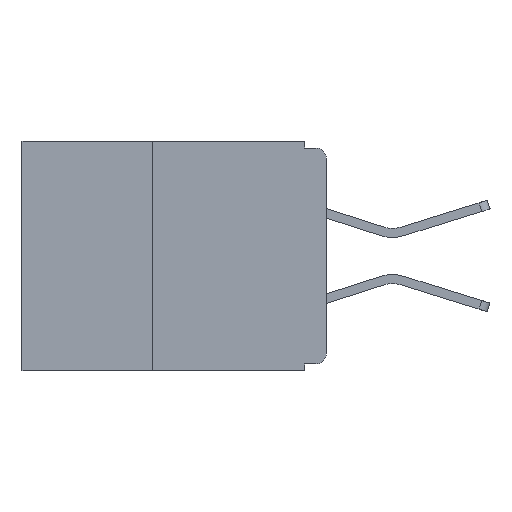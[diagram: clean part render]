
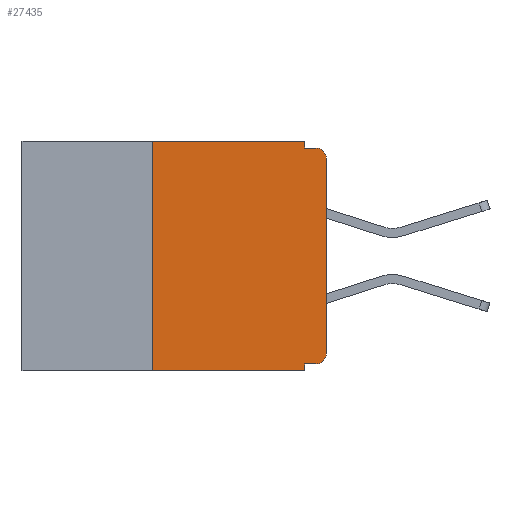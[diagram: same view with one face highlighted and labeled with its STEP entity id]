
A CAD part, left-side view. The second image highlights one B-rep face of the part: STEP entity #27435.
In plain terms, the highlighted planar face has unit normal (-1, 0, 0).
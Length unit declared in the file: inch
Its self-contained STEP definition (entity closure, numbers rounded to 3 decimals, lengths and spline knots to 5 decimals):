
#333 = VECTOR ( 'NONE', #11495, 39.37008 ) ;
#669 = CARTESIAN_POINT ( 'NONE',  ( 0., 0.031, -0.33 ) ) ;
#891 = LINE ( 'NONE', #5456, #17757 ) ;
#1060 = DIRECTION ( 'NONE',  ( 0., 0., -1. ) ) ;
#1680 = ORIENTED_EDGE ( 'NONE', *, *, #9738, .T. ) ;
#1788 = DIRECTION ( 'NONE',  ( 1., 0., 0. ) ) ;
#2608 = LINE ( 'NONE', #24491, #7786 ) ;
#2718 = ORIENTED_EDGE ( 'NONE', *, *, #19798, .T. ) ;
#3532 = DIRECTION ( 'NONE',  ( -1., 0., 0. ) ) ;
#3645 = LINE ( 'NONE', #22885, #8799 ) ;
#3854 = EDGE_CURVE ( 'NONE', #20469, #16692, #12098, .T. ) ;
#4030 = VECTOR ( 'NONE', #11167, 39.37008 ) ;
#4216 = VERTEX_POINT ( 'NONE', #9348 ) ;
#4595 = CARTESIAN_POINT ( 'NONE',  ( 0., 0., -0.01 ) ) ;
#4618 = EDGE_CURVE ( 'NONE', #8001, #8071, #25678, .T. ) ;
#4669 = VECTOR ( 'NONE', #8589, 39.37008 ) ;
#5195 = DIRECTION ( 'NONE',  ( 0., 0., 1. ) ) ;
#5456 = CARTESIAN_POINT ( 'NONE',  ( 0., 0.031, 0. ) ) ;
#5516 = ORIENTED_EDGE ( 'NONE', *, *, #13326, .F. ) ;
#6129 = CARTESIAN_POINT ( 'NONE',  ( 0., 0.25, 0. ) ) ;
#6746 = CARTESIAN_POINT ( 'NONE',  ( 0., 0.437, -0.33 ) ) ;
#7203 = DIRECTION ( 'NONE',  ( -1., 0., 0. ) ) ;
#7786 = VECTOR ( 'NONE', #9240, 39.37008 ) ;
#7868 = VERTEX_POINT ( 'NONE', #13543 ) ;
#7891 = ORIENTED_EDGE ( 'NONE', *, *, #13430, .T. ) ;
#8001 = VERTEX_POINT ( 'NONE', #13922 ) ;
#8071 = VERTEX_POINT ( 'NONE', #18482 ) ;
#8134 = CARTESIAN_POINT ( 'NONE',  ( 0., 0.25, -0.33 ) ) ;
#8349 = CARTESIAN_POINT ( 'NONE',  ( 0., 0.437, 0. ) ) ;
#8589 = DIRECTION ( 'NONE',  ( 0., 0., 1. ) ) ;
#8799 = VECTOR ( 'NONE', #9829, 39.37008 ) ;
#9240 = DIRECTION ( 'NONE',  ( 0., -1., 0. ) ) ;
#9348 = CARTESIAN_POINT ( 'NONE',  ( 0., 0.031, 0. ) ) ;
#9738 = EDGE_CURVE ( 'NONE', #26208, #16692, #9860, .T. ) ;
#9829 = DIRECTION ( 'NONE',  ( 0., 1., 0. ) ) ;
#9860 = LINE ( 'NONE', #6746, #4030 ) ;
#11008 = CARTESIAN_POINT ( 'NONE',  ( 0., 0., -0.305 ) ) ;
#11167 = DIRECTION ( 'NONE',  ( 0., -1., 0. ) ) ;
#11206 = LINE ( 'NONE', #12996, #4669 ) ;
#11226 = EDGE_CURVE ( 'NONE', #26208, #14299, #11206, .T. ) ;
#11495 = DIRECTION ( 'NONE',  ( 0., 0., -1. ) ) ;
#11902 = CARTESIAN_POINT ( 'NONE',  ( 0., 0.031, -0.33 ) ) ;
#12098 = LINE ( 'NONE', #11902, #333 ) ;
#12512 = VERTEX_POINT ( 'NONE', #13694 ) ;
#12675 = EDGE_CURVE ( 'NONE', #4216, #8001, #891, .T. ) ;
#12759 = PLANE ( 'NONE',  #18328 ) ;
#12930 = LINE ( 'NONE', #22648, #22460 ) ;
#12996 = CARTESIAN_POINT ( 'NONE',  ( 0., 0.25, -0.33 ) ) ;
#13326 = EDGE_CURVE ( 'NONE', #14299, #4216, #2608, .T. ) ;
#13430 = EDGE_CURVE ( 'NONE', #27715, #7868, #12930, .T. ) ;
#13543 = CARTESIAN_POINT ( 'NONE',  ( 0., 0., -0.025 ) ) ;
#13694 = CARTESIAN_POINT ( 'NONE',  ( 0., 0.015, -0.32 ) ) ;
#13922 = CARTESIAN_POINT ( 'NONE',  ( 0., 0.031, -0.01 ) ) ;
#14077 = ORIENTED_EDGE ( 'NONE', *, *, #3854, .F. ) ;
#14299 = VERTEX_POINT ( 'NONE', #6129 ) ;
#14477 = AXIS2_PLACEMENT_3D ( 'NONE', #16644, #3532, #18835 ) ;
#14790 = ORIENTED_EDGE ( 'NONE', *, *, #24220, .F. ) ;
#15472 = EDGE_CURVE ( 'NONE', #12512, #27715, #28146, .T. ) ;
#16184 = EDGE_LOOP ( 'NONE', ( #7891, #2718, #20852, #22236, #5516, #17832, #1680, #14077, #14790, #26337 ) ) ;
#16644 = CARTESIAN_POINT ( 'NONE',  ( 0., 0.015, -0.305 ) ) ;
#16692 = VERTEX_POINT ( 'NONE', #669 ) ;
#17136 = DIRECTION ( 'NONE',  ( 0., 0., -1. ) ) ;
#17757 = VECTOR ( 'NONE', #1060, 39.37008 ) ;
#17832 = ORIENTED_EDGE ( 'NONE', *, *, #11226, .F. ) ;
#18328 = AXIS2_PLACEMENT_3D ( 'NONE', #8349, #1788, #17136 ) ;
#18482 = CARTESIAN_POINT ( 'NONE',  ( 0., 0.015, -0.01 ) ) ;
#18835 = DIRECTION ( 'NONE',  ( 0., 0., -1. ) ) ;
#19798 = EDGE_CURVE ( 'NONE', #7868, #8071, #20266, .T. ) ;
#19867 = DIRECTION ( 'NONE',  ( 0., -1., 0. ) ) ;
#20059 = FACE_OUTER_BOUND ( 'NONE', #16184, .T. ) ;
#20261 = CARTESIAN_POINT ( 'NONE',  ( 0., 0.015, -0.025 ) ) ;
#20266 = CIRCLE ( 'NONE', #26737, 0.015 ) ;
#20469 = VERTEX_POINT ( 'NONE', #26905 ) ;
#20549 = VECTOR ( 'NONE', #19867, 39.37008 ) ;
#20852 = ORIENTED_EDGE ( 'NONE', *, *, #4618, .F. ) ;
#22236 = ORIENTED_EDGE ( 'NONE', *, *, #12675, .F. ) ;
#22458 = DIRECTION ( 'NONE',  ( 0., 0., -1. ) ) ;
#22460 = VECTOR ( 'NONE', #5195, 39.37008 ) ;
#22648 = CARTESIAN_POINT ( 'NONE',  ( 0., 0., 0. ) ) ;
#22885 = CARTESIAN_POINT ( 'NONE',  ( 0., 0., -0.32 ) ) ;
#24220 = EDGE_CURVE ( 'NONE', #12512, #20469, #3645, .T. ) ;
#24491 = CARTESIAN_POINT ( 'NONE',  ( 0., 0.437, 0. ) ) ;
#25678 = LINE ( 'NONE', #4595, #20549 ) ;
#26208 = VERTEX_POINT ( 'NONE', #8134 ) ;
#26337 = ORIENTED_EDGE ( 'NONE', *, *, #15472, .T. ) ;
#26737 = AXIS2_PLACEMENT_3D ( 'NONE', #20261, #7203, #22458 ) ;
#26905 = CARTESIAN_POINT ( 'NONE',  ( 0., 0.031, -0.32 ) ) ;
#27435 = ADVANCED_FACE ( 'NONE', ( #20059 ), #12759, .F. ) ;
#27715 = VERTEX_POINT ( 'NONE', #11008 ) ;
#28146 = CIRCLE ( 'NONE', #14477, 0.015 ) ;
